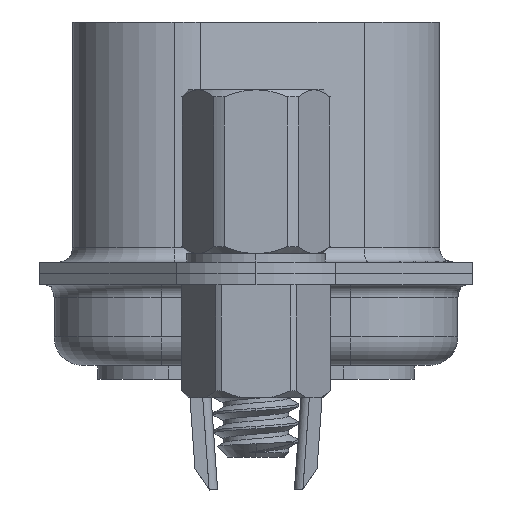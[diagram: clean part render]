
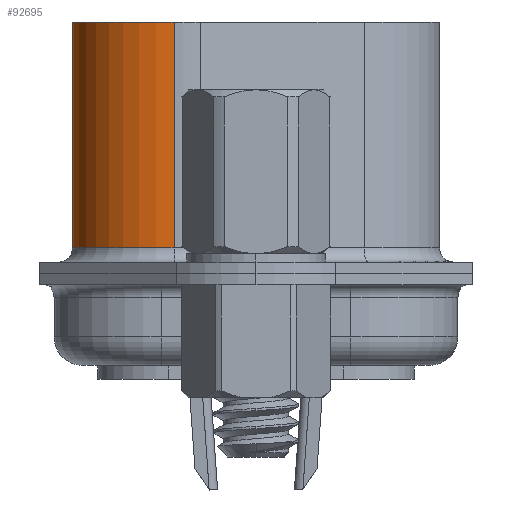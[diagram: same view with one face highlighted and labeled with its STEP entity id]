
A CAD part, left-side view. The second image highlights one B-rep face of the part: STEP entity #92695.
In plain terms, the highlighted cylindrical face has radius 3.6 mm (diameter 7.2 mm), a partial arc.
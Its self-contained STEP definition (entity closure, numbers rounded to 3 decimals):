
#7899 = LINE ( 'NONE', #171152, #137448 ) ;
#14638 = CARTESIAN_POINT ( 'NONE',  ( 8.39, 2.9, 9.3 ) ) ;
#20229 = ORIENTED_EDGE ( 'NONE', *, *, #163790, .F. ) ;
#22718 = VERTEX_POINT ( 'NONE', #95465 ) ;
#28957 = VERTEX_POINT ( 'NONE', #130412 ) ;
#33914 = EDGE_CURVE ( 'NONE', #22718, #28957, #121750, .T. ) ;
#35075 = DIRECTION ( 'NONE',  ( -1., 0., 0. ) ) ;
#39491 = CARTESIAN_POINT ( 'NONE',  ( 8.39, 2.9, 9.3 ) ) ;
#50443 = VERTEX_POINT ( 'NONE', #164868 ) ;
#66987 = DIRECTION ( 'NONE',  ( 0., 0., -1. ) ) ;
#69987 = AXIS2_PLACEMENT_3D ( 'NONE', #14638, #152155, #96288 ) ;
#73008 = ORIENTED_EDGE ( 'NONE', *, *, #33914, .T. ) ;
#74992 = CARTESIAN_POINT ( 'NONE',  ( 8.39, 2.9, 1.3 ) ) ;
#80031 = VERTEX_POINT ( 'NONE', #132965 ) ;
#84159 = CIRCLE ( 'NONE', #69987, 3.6 ) ;
#89505 = DIRECTION ( 'NONE',  ( 0., 0., -1. ) ) ;
#92695 = ADVANCED_FACE ( 'NONE', ( #146890 ), #146021, .T. ) ;
#95465 = CARTESIAN_POINT ( 'NONE',  ( 8.39, 6.5, 1.3 ) ) ;
#96288 = DIRECTION ( 'NONE',  ( 1., 0., 0. ) ) ;
#116144 = AXIS2_PLACEMENT_3D ( 'NONE', #74992, #140751, #35075 ) ;
#121068 = AXIS2_PLACEMENT_3D ( 'NONE', #39491, #66987, #162835 ) ;
#121428 = LINE ( 'NONE', #144750, #132888 ) ;
#121750 = CIRCLE ( 'NONE', #116144, 3.6 ) ;
#125828 = EDGE_LOOP ( 'NONE', ( #147429, #20229, #134220, #73008 ) ) ;
#130412 = CARTESIAN_POINT ( 'NONE',  ( 4.79, 2.9, 1.3 ) ) ;
#132888 = VECTOR ( 'NONE', #175553, 1000. ) ;
#132965 = CARTESIAN_POINT ( 'NONE',  ( 4.79, 2.9, 9.3 ) ) ;
#134220 = ORIENTED_EDGE ( 'NONE', *, *, #156368, .T. ) ;
#137448 = VECTOR ( 'NONE', #89505, 1000. ) ;
#140751 = DIRECTION ( 'NONE',  ( 0., 0., 1. ) ) ;
#144750 = CARTESIAN_POINT ( 'NONE',  ( 8.39, 6.5, 9.3 ) ) ;
#146021 = CYLINDRICAL_SURFACE ( 'NONE', #121068, 3.6 ) ;
#146890 = FACE_OUTER_BOUND ( 'NONE', #125828, .T. ) ;
#147429 = ORIENTED_EDGE ( 'NONE', *, *, #159846, .F. ) ;
#152155 = DIRECTION ( 'NONE',  ( 0., 0., 1. ) ) ;
#156368 = EDGE_CURVE ( 'NONE', #50443, #22718, #121428, .T. ) ;
#159846 = EDGE_CURVE ( 'NONE', #80031, #28957, #7899, .T. ) ;
#162835 = DIRECTION ( 'NONE',  ( -1., 0., 0. ) ) ;
#163790 = EDGE_CURVE ( 'NONE', #50443, #80031, #84159, .T. ) ;
#164868 = CARTESIAN_POINT ( 'NONE',  ( 8.39, 6.5, 9.3 ) ) ;
#171152 = CARTESIAN_POINT ( 'NONE',  ( 4.79, 2.9, 9.3 ) ) ;
#175553 = DIRECTION ( 'NONE',  ( 0., 0., -1. ) ) ;
